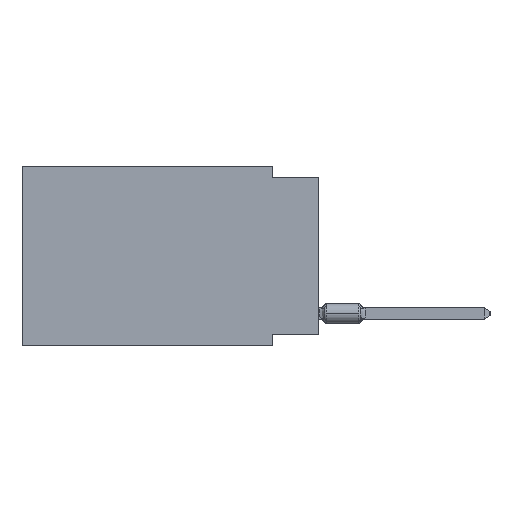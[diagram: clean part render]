
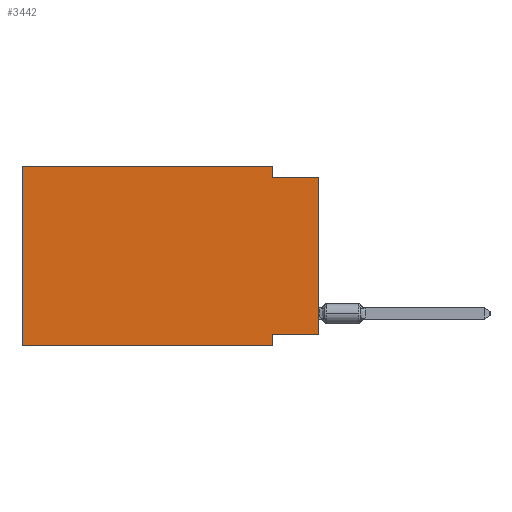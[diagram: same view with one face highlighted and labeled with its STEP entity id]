
A CAD part, left-side view. The second image highlights one B-rep face of the part: STEP entity #3442.
In plain terms, the highlighted planar face has unit normal (-1, 0, 0).
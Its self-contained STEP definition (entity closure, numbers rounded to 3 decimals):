
#95 = EDGE_CURVE ( 'NONE', #29018, #10575, #29170, .T. ) ;
#488 = DIRECTION ( 'NONE',  ( 0., 0., 1. ) ) ;
#682 = EDGE_CURVE ( 'NONE', #27084, #8285, #10778, .T. ) ;
#1712 = VECTOR ( 'NONE', #488, 1000. ) ;
#1847 = DIRECTION ( 'NONE',  ( 0., -1., 0. ) ) ;
#2156 = VECTOR ( 'NONE', #28739, 1000. ) ;
#2264 = EDGE_CURVE ( 'NONE', #26793, #10575, #9707, .T. ) ;
#2974 = ORIENTED_EDGE ( 'NONE', *, *, #682, .F. ) ;
#3442 = ADVANCED_FACE ( 'NONE', ( #4192 ), #9108, .F. ) ;
#4192 = FACE_OUTER_BOUND ( 'NONE', #20449, .T. ) ;
#5917 = CARTESIAN_POINT ( 'NONE',  ( 0., 2.54, -9.271 ) ) ;
#6075 = ORIENTED_EDGE ( 'NONE', *, *, #2264, .T. ) ;
#6206 = CARTESIAN_POINT ( 'NONE',  ( 0., 0., -0.635 ) ) ;
#6842 = CARTESIAN_POINT ( 'NONE',  ( 0., 2.54, 0. ) ) ;
#7216 = DIRECTION ( 'NONE',  ( 0., 1., 0. ) ) ;
#8285 = VERTEX_POINT ( 'NONE', #29313 ) ;
#9108 = PLANE ( 'NONE',  #17705 ) ;
#9129 = EDGE_CURVE ( 'NONE', #16889, #8285, #23595, .T. ) ;
#9437 = ORIENTED_EDGE ( 'NONE', *, *, #9129, .T. ) ;
#9540 = DIRECTION ( 'NONE',  ( 0., -1., 0. ) ) ;
#9707 = LINE ( 'NONE', #24882, #27955 ) ;
#10492 = VERTEX_POINT ( 'NONE', #6842 ) ;
#10575 = VERTEX_POINT ( 'NONE', #11908 ) ;
#10778 = LINE ( 'NONE', #6206, #30549 ) ;
#10864 = CARTESIAN_POINT ( 'NONE',  ( 0., 16.383, 0. ) ) ;
#11798 = DIRECTION ( 'NONE',  ( 0., 0., -1. ) ) ;
#11908 = CARTESIAN_POINT ( 'NONE',  ( 0., 2.54, -9.906 ) ) ;
#11942 = EDGE_CURVE ( 'NONE', #16889, #29018, #20191, .T. ) ;
#12499 = EDGE_CURVE ( 'NONE', #10492, #27084, #20626, .T. ) ;
#13150 = EDGE_CURVE ( 'NONE', #16759, #10492, #27661, .T. ) ;
#13281 = VECTOR ( 'NONE', #18706, 1000. ) ;
#13414 = ORIENTED_EDGE ( 'NONE', *, *, #95, .F. ) ;
#13482 = DIRECTION ( 'NONE',  ( 0., -1., 0. ) ) ;
#14327 = DIRECTION ( 'NONE',  ( 1., 0., 0. ) ) ;
#15147 = CARTESIAN_POINT ( 'NONE',  ( 0., 0., -9.271 ) ) ;
#15920 = CARTESIAN_POINT ( 'NONE',  ( 0., 2.54, 0. ) ) ;
#16759 = VERTEX_POINT ( 'NONE', #32001 ) ;
#16889 = VERTEX_POINT ( 'NONE', #25397 ) ;
#17201 = CARTESIAN_POINT ( 'NONE',  ( 0., 16.383, 0. ) ) ;
#17705 = AXIS2_PLACEMENT_3D ( 'NONE', #24940, #14327, #11798 ) ;
#18706 = DIRECTION ( 'NONE',  ( 0., 0., -1. ) ) ;
#20191 = LINE ( 'NONE', #15147, #32641 ) ;
#20449 = EDGE_LOOP ( 'NONE', ( #9437, #2974, #22348, #31899, #29574, #6075, #13414, #22590 ) ) ;
#20626 = LINE ( 'NONE', #15920, #26700 ) ;
#21736 = CARTESIAN_POINT ( 'NONE',  ( 0., 2.54, -9.906 ) ) ;
#22348 = ORIENTED_EDGE ( 'NONE', *, *, #12499, .F. ) ;
#22590 = ORIENTED_EDGE ( 'NONE', *, *, #11942, .F. ) ;
#23595 = LINE ( 'NONE', #28339, #1712 ) ;
#24882 = CARTESIAN_POINT ( 'NONE',  ( 0., 16.383, -9.906 ) ) ;
#24940 = CARTESIAN_POINT ( 'NONE',  ( 0., 16.383, 0. ) ) ;
#25397 = CARTESIAN_POINT ( 'NONE',  ( 0., 0., -9.271 ) ) ;
#26700 = VECTOR ( 'NONE', #31094, 1000. ) ;
#26793 = VERTEX_POINT ( 'NONE', #32500 ) ;
#27084 = VERTEX_POINT ( 'NONE', #28608 ) ;
#27661 = LINE ( 'NONE', #17201, #31130 ) ;
#27955 = VECTOR ( 'NONE', #9540, 1000. ) ;
#28339 = CARTESIAN_POINT ( 'NONE',  ( 0., 0., 0. ) ) ;
#28608 = CARTESIAN_POINT ( 'NONE',  ( 0., 2.54, -0.635 ) ) ;
#28739 = DIRECTION ( 'NONE',  ( 0., 0., 1. ) ) ;
#29018 = VERTEX_POINT ( 'NONE', #5917 ) ;
#29085 = LINE ( 'NONE', #10864, #2156 ) ;
#29170 = LINE ( 'NONE', #21736, #13281 ) ;
#29313 = CARTESIAN_POINT ( 'NONE',  ( 0., 0., -0.635 ) ) ;
#29574 = ORIENTED_EDGE ( 'NONE', *, *, #31083, .F. ) ;
#30549 = VECTOR ( 'NONE', #13482, 1000. ) ;
#31083 = EDGE_CURVE ( 'NONE', #26793, #16759, #29085, .T. ) ;
#31094 = DIRECTION ( 'NONE',  ( 0., 0., -1. ) ) ;
#31130 = VECTOR ( 'NONE', #1847, 1000. ) ;
#31899 = ORIENTED_EDGE ( 'NONE', *, *, #13150, .F. ) ;
#32001 = CARTESIAN_POINT ( 'NONE',  ( 0., 16.383, 0. ) ) ;
#32500 = CARTESIAN_POINT ( 'NONE',  ( 0., 16.383, -9.906 ) ) ;
#32641 = VECTOR ( 'NONE', #7216, 1000. ) ;
